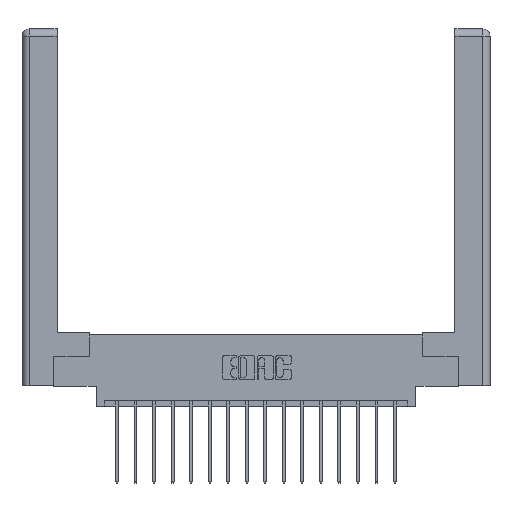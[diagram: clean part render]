
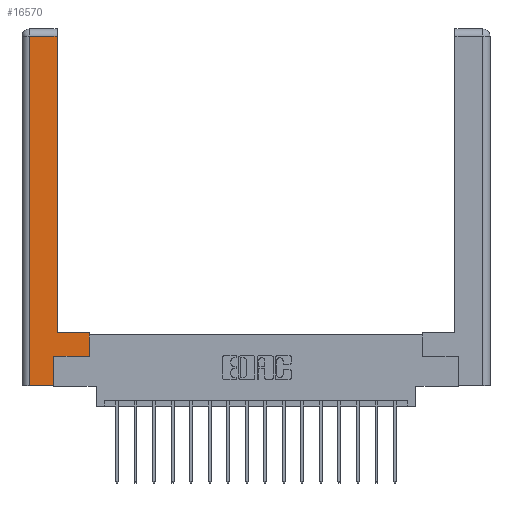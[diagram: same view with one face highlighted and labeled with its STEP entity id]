
A CAD part, top view. The second image highlights one B-rep face of the part: STEP entity #16570.
In plain terms, the highlighted planar face has unit normal (0, 0, 1).
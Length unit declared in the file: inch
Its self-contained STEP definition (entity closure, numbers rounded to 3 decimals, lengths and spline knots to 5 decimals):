
#182 = DIRECTION ( 'NONE',  ( 1., 0., 0. ) ) ;
#577 = VECTOR ( 'NONE', #3229, 39.37008 ) ;
#752 = CARTESIAN_POINT ( 'NONE',  ( 0., 0., 0. ) ) ;
#1352 = VERTEX_POINT ( 'NONE', #11414 ) ;
#1870 = CARTESIAN_POINT ( 'NONE',  ( 0.265, 0.245, 0. ) ) ;
#2266 = VECTOR ( 'NONE', #6495, 39.37008 ) ;
#2488 = CARTESIAN_POINT ( 'NONE',  ( 0.0615, 0., 0. ) ) ;
#2546 = VERTEX_POINT ( 'NONE', #18350 ) ;
#2711 = LINE ( 'NONE', #1870, #12584 ) ;
#2975 = CARTESIAN_POINT ( 'NONE',  ( 0.295, 0.45, 0. ) ) ;
#3229 = DIRECTION ( 'NONE',  ( 0., 1., 0. ) ) ;
#3735 = VECTOR ( 'NONE', #13526, 39.37008 ) ;
#3777 = DIRECTION ( 'NONE',  ( 0., 1., 0. ) ) ;
#3809 = CARTESIAN_POINT ( 'NONE',  ( 0.565, 0.245, 0. ) ) ;
#3940 = DIRECTION ( 'NONE',  ( 0., -1., 0. ) ) ;
#4160 = EDGE_CURVE ( 'NONE', #6791, #10492, #14165, .T. ) ;
#4398 = ORIENTED_EDGE ( 'NONE', *, *, #8179, .T. ) ;
#5088 = VECTOR ( 'NONE', #10672, 39.37008 ) ;
#5730 = CARTESIAN_POINT ( 'NONE',  ( 0.0615, 2.94, 0. ) ) ;
#6207 = LINE ( 'NONE', #16399, #3735 ) ;
#6230 = ORIENTED_EDGE ( 'NONE', *, *, #18045, .T. ) ;
#6495 = DIRECTION ( 'NONE',  ( 1., 0., 0. ) ) ;
#6791 = VERTEX_POINT ( 'NONE', #7267 ) ;
#6808 = VERTEX_POINT ( 'NONE', #5730 ) ;
#7063 = VECTOR ( 'NONE', #3940, 39.37008 ) ;
#7099 = EDGE_CURVE ( 'NONE', #12712, #6808, #6207, .T. ) ;
#7135 = EDGE_CURVE ( 'NONE', #10492, #13866, #14263, .T. ) ;
#7267 = CARTESIAN_POINT ( 'NONE',  ( 0.265, 0.245, 0. ) ) ;
#7508 = LINE ( 'NONE', #2488, #7063 ) ;
#7876 = EDGE_CURVE ( 'NONE', #6808, #1352, #7508, .T. ) ;
#8179 = EDGE_CURVE ( 'NONE', #14724, #12712, #8853, .T. ) ;
#8431 = EDGE_CURVE ( 'NONE', #1352, #2546, #11761, .T. ) ;
#8606 = EDGE_LOOP ( 'NONE', ( #4398, #12728, #13498, #15417, #6230, #15762, #14665, #10933 ) ) ;
#8853 = LINE ( 'NONE', #11800, #577 ) ;
#10492 = VERTEX_POINT ( 'NONE', #12284 ) ;
#10672 = DIRECTION ( 'NONE',  ( -1., 0., 0. ) ) ;
#10933 = ORIENTED_EDGE ( 'NONE', *, *, #11538, .T. ) ;
#11414 = CARTESIAN_POINT ( 'NONE',  ( 0.0615, 0., 0. ) ) ;
#11538 = EDGE_CURVE ( 'NONE', #13866, #14724, #11784, .T. ) ;
#11637 = CARTESIAN_POINT ( 'NONE',  ( 0.265, 0., 0. ) ) ;
#11761 = LINE ( 'NONE', #11637, #18294 ) ;
#11784 = LINE ( 'NONE', #13235, #5088 ) ;
#11800 = CARTESIAN_POINT ( 'NONE',  ( 0.295, 3., 0. ) ) ;
#11869 = DIRECTION ( 'NONE',  ( 0., 1., 0. ) ) ;
#12237 = CARTESIAN_POINT ( 'NONE',  ( 0.565, 0.45, 0. ) ) ;
#12268 = DIRECTION ( 'NONE',  ( -1., 0., 0. ) ) ;
#12284 = CARTESIAN_POINT ( 'NONE',  ( 0.565, 0.245, 0. ) ) ;
#12584 = VECTOR ( 'NONE', #11869, 39.37008 ) ;
#12712 = VERTEX_POINT ( 'NONE', #14094 ) ;
#12728 = ORIENTED_EDGE ( 'NONE', *, *, #7099, .T. ) ;
#13097 = AXIS2_PLACEMENT_3D ( 'NONE', #752, #13589, #12268 ) ;
#13235 = CARTESIAN_POINT ( 'NONE',  ( 0.295, 0.45, 0. ) ) ;
#13498 = ORIENTED_EDGE ( 'NONE', *, *, #7876, .T. ) ;
#13526 = DIRECTION ( 'NONE',  ( -1., 0., 0. ) ) ;
#13589 = DIRECTION ( 'NONE',  ( 0., 0., -1. ) ) ;
#13754 = FACE_OUTER_BOUND ( 'NONE', #8606, .T. ) ;
#13866 = VERTEX_POINT ( 'NONE', #12237 ) ;
#14094 = CARTESIAN_POINT ( 'NONE',  ( 0.295, 2.94, 0. ) ) ;
#14165 = LINE ( 'NONE', #3809, #2266 ) ;
#14263 = LINE ( 'NONE', #18246, #17875 ) ;
#14665 = ORIENTED_EDGE ( 'NONE', *, *, #7135, .T. ) ;
#14724 = VERTEX_POINT ( 'NONE', #2975 ) ;
#15417 = ORIENTED_EDGE ( 'NONE', *, *, #8431, .T. ) ;
#15762 = ORIENTED_EDGE ( 'NONE', *, *, #4160, .T. ) ;
#16399 = CARTESIAN_POINT ( 'NONE',  ( 0.0615, 2.94, 0. ) ) ;
#16570 = ADVANCED_FACE ( 'NONE', ( #13754 ), #17945, .F. ) ;
#17875 = VECTOR ( 'NONE', #3777, 39.37008 ) ;
#17945 = PLANE ( 'NONE',  #13097 ) ;
#18045 = EDGE_CURVE ( 'NONE', #2546, #6791, #2711, .T. ) ;
#18246 = CARTESIAN_POINT ( 'NONE',  ( 0.565, 0.45, 0. ) ) ;
#18294 = VECTOR ( 'NONE', #182, 39.37008 ) ;
#18350 = CARTESIAN_POINT ( 'NONE',  ( 0.265, 0., 0. ) ) ;
